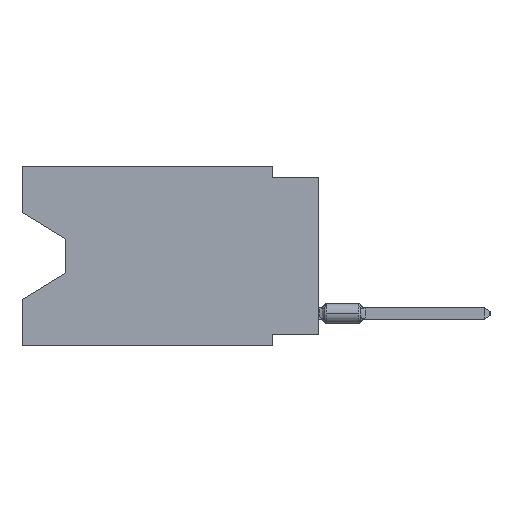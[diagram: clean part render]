
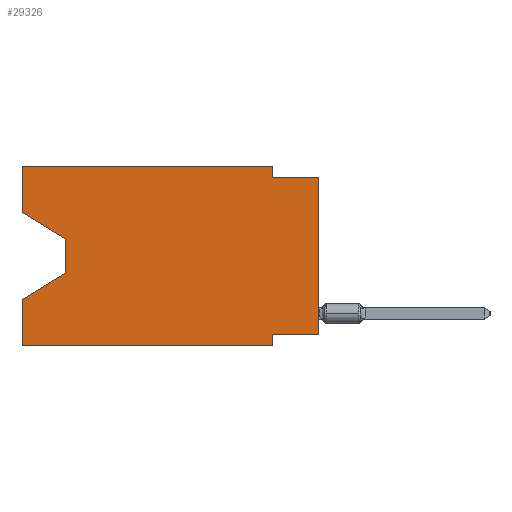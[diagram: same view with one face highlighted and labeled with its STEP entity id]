
A CAD part, left-side view. The second image highlights one B-rep face of the part: STEP entity #29326.
In plain terms, the highlighted planar face has unit normal (-1, 0, 0).
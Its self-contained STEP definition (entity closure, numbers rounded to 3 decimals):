
#378 = EDGE_CURVE ( 'NONE', #15556, #2593, #25521, .T. ) ;
#432 = CARTESIAN_POINT ( 'NONE',  ( 0., 2.54, 0. ) ) ;
#511 = ORIENTED_EDGE ( 'NONE', *, *, #27226, .F. ) ;
#1447 = DIRECTION ( 'NONE',  ( 0., 1., 0. ) ) ;
#1590 = DIRECTION ( 'NONE',  ( 0., 0., 1. ) ) ;
#1791 = DIRECTION ( 'NONE',  ( 0., -0.855, -0.519 ) ) ;
#1927 = CARTESIAN_POINT ( 'NONE',  ( 0., 2.54, -9.906 ) ) ;
#2593 = VERTEX_POINT ( 'NONE', #32092 ) ;
#2703 = VECTOR ( 'NONE', #1590, 1000. ) ;
#3058 = DIRECTION ( 'NONE',  ( 0., 0.855, -0.519 ) ) ;
#3186 = VERTEX_POINT ( 'NONE', #12722 ) ;
#3612 = EDGE_CURVE ( 'NONE', #22711, #16617, #22225, .T. ) ;
#4272 = DIRECTION ( 'NONE',  ( 1., 0., 0. ) ) ;
#4531 = CARTESIAN_POINT ( 'NONE',  ( 0., 0., 0. ) ) ;
#5199 = CARTESIAN_POINT ( 'NONE',  ( 0., 16.383, -7.36 ) ) ;
#5386 = DIRECTION ( 'NONE',  ( 0., 0., 1. ) ) ;
#5462 = DIRECTION ( 'NONE',  ( 0., -1., 0. ) ) ;
#5693 = DIRECTION ( 'NONE',  ( 0., -1., 0. ) ) ;
#6014 = LINE ( 'NONE', #6197, #28349 ) ;
#6197 = CARTESIAN_POINT ( 'NONE',  ( 0., 16.383, 0. ) ) ;
#6799 = EDGE_CURVE ( 'NONE', #3186, #20952, #14919, .T. ) ;
#7032 = FACE_OUTER_BOUND ( 'NONE', #18373, .T. ) ;
#7128 = ORIENTED_EDGE ( 'NONE', *, *, #35729, .T. ) ;
#7172 = ORIENTED_EDGE ( 'NONE', *, *, #3612, .T. ) ;
#7250 = CARTESIAN_POINT ( 'NONE',  ( 0., 2.54, 0. ) ) ;
#8237 = VERTEX_POINT ( 'NONE', #22842 ) ;
#8382 = LINE ( 'NONE', #17988, #21376 ) ;
#8900 = ORIENTED_EDGE ( 'NONE', *, *, #30977, .F. ) ;
#9232 = CARTESIAN_POINT ( 'NONE',  ( 0., 16.383, -9.906 ) ) ;
#9713 = ORIENTED_EDGE ( 'NONE', *, *, #31710, .F. ) ;
#11893 = VECTOR ( 'NONE', #5386, 1000. ) ;
#12301 = ORIENTED_EDGE ( 'NONE', *, *, #6799, .T. ) ;
#12355 = EDGE_CURVE ( 'NONE', #22711, #8237, #37967, .T. ) ;
#12722 = CARTESIAN_POINT ( 'NONE',  ( 0., 16.383, -9.906 ) ) ;
#13727 = CARTESIAN_POINT ( 'NONE',  ( 0., 16.383, -2.546 ) ) ;
#14317 = CARTESIAN_POINT ( 'NONE',  ( 0., 13.97, -4.013 ) ) ;
#14728 = CARTESIAN_POINT ( 'NONE',  ( 0., 13.97, -5.893 ) ) ;
#14842 = DIRECTION ( 'NONE',  ( 0., 0., 1. ) ) ;
#14919 = LINE ( 'NONE', #9232, #26796 ) ;
#15556 = VERTEX_POINT ( 'NONE', #432 ) ;
#15657 = VERTEX_POINT ( 'NONE', #13727 ) ;
#16235 = DIRECTION ( 'NONE',  ( 0., 0., -1. ) ) ;
#16363 = DIRECTION ( 'NONE',  ( 0., 0., -1. ) ) ;
#16617 = VERTEX_POINT ( 'NONE', #36670 ) ;
#16864 = EDGE_CURVE ( 'NONE', #15657, #26306, #34035, .T. ) ;
#17988 = CARTESIAN_POINT ( 'NONE',  ( 0., 13.97, -5.893 ) ) ;
#18373 = EDGE_LOOP ( 'NONE', ( #22738, #33115, #7128, #20148, #12301, #9713, #18782, #7172, #23808, #25670, #8900, #511 ) ) ;
#18782 = ORIENTED_EDGE ( 'NONE', *, *, #12355, .F. ) ;
#20148 = ORIENTED_EDGE ( 'NONE', *, *, #24530, .F. ) ;
#20176 = LINE ( 'NONE', #32192, #31609 ) ;
#20952 = VERTEX_POINT ( 'NONE', #1927 ) ;
#21231 = VECTOR ( 'NONE', #1791, 1000. ) ;
#21332 = VECTOR ( 'NONE', #16363, 1000. ) ;
#21376 = VECTOR ( 'NONE', #3058, 1000. ) ;
#21600 = LINE ( 'NONE', #34171, #30300 ) ;
#22225 = LINE ( 'NONE', #4531, #2703 ) ;
#22711 = VERTEX_POINT ( 'NONE', #27203 ) ;
#22738 = ORIENTED_EDGE ( 'NONE', *, *, #16864, .T. ) ;
#22842 = CARTESIAN_POINT ( 'NONE',  ( 0., 2.54, -9.271 ) ) ;
#23808 = ORIENTED_EDGE ( 'NONE', *, *, #28529, .F. ) ;
#24530 = EDGE_CURVE ( 'NONE', #3186, #37395, #31901, .T. ) ;
#24847 = DIRECTION ( 'NONE',  ( 0., 0., -1. ) ) ;
#24944 = DIRECTION ( 'NONE',  ( 0., -1., 0. ) ) ;
#25365 = EDGE_CURVE ( 'NONE', #26306, #30539, #25628, .T. ) ;
#25432 = LINE ( 'NONE', #37398, #36014 ) ;
#25521 = LINE ( 'NONE', #7250, #26675 ) ;
#25628 = LINE ( 'NONE', #28193, #21332 ) ;
#25670 = ORIENTED_EDGE ( 'NONE', *, *, #378, .F. ) ;
#25892 = PLANE ( 'NONE',  #31612 ) ;
#25920 = VECTOR ( 'NONE', #1447, 1000. ) ;
#26306 = VERTEX_POINT ( 'NONE', #14317 ) ;
#26675 = VECTOR ( 'NONE', #33767, 1000. ) ;
#26796 = VECTOR ( 'NONE', #5693, 1000. ) ;
#27203 = CARTESIAN_POINT ( 'NONE',  ( 0., 0., -9.271 ) ) ;
#27226 = EDGE_CURVE ( 'NONE', #15657, #35727, #6014, .T. ) ;
#28193 = CARTESIAN_POINT ( 'NONE',  ( 0., 13.97, -4.013 ) ) ;
#28349 = VECTOR ( 'NONE', #14842, 1000. ) ;
#28361 = CARTESIAN_POINT ( 'NONE',  ( 0., 0., -9.271 ) ) ;
#28529 = EDGE_CURVE ( 'NONE', #2593, #16617, #21600, .T. ) ;
#29326 = ADVANCED_FACE ( 'NONE', ( #7032 ), #25892, .F. ) ;
#30300 = VECTOR ( 'NONE', #24944, 1000. ) ;
#30539 = VERTEX_POINT ( 'NONE', #14728 ) ;
#30977 = EDGE_CURVE ( 'NONE', #35727, #15556, #20176, .T. ) ;
#31212 = CARTESIAN_POINT ( 'NONE',  ( 0., 16.383, 0. ) ) ;
#31471 = CARTESIAN_POINT ( 'NONE',  ( 0., 16.383, -2.546 ) ) ;
#31609 = VECTOR ( 'NONE', #5462, 1000. ) ;
#31612 = AXIS2_PLACEMENT_3D ( 'NONE', #31212, #4272, #16235 ) ;
#31710 = EDGE_CURVE ( 'NONE', #8237, #20952, #25432, .T. ) ;
#31901 = LINE ( 'NONE', #32316, #11893 ) ;
#32092 = CARTESIAN_POINT ( 'NONE',  ( 0., 2.54, -0.635 ) ) ;
#32192 = CARTESIAN_POINT ( 'NONE',  ( 0., 16.383, 0. ) ) ;
#32316 = CARTESIAN_POINT ( 'NONE',  ( 0., 16.383, 0. ) ) ;
#32541 = CARTESIAN_POINT ( 'NONE',  ( 0., 16.383, 0. ) ) ;
#33115 = ORIENTED_EDGE ( 'NONE', *, *, #25365, .T. ) ;
#33767 = DIRECTION ( 'NONE',  ( 0., 0., -1. ) ) ;
#34035 = LINE ( 'NONE', #31471, #21231 ) ;
#34171 = CARTESIAN_POINT ( 'NONE',  ( 0., 0., -0.635 ) ) ;
#35727 = VERTEX_POINT ( 'NONE', #32541 ) ;
#35729 = EDGE_CURVE ( 'NONE', #30539, #37395, #8382, .T. ) ;
#36014 = VECTOR ( 'NONE', #24847, 1000. ) ;
#36670 = CARTESIAN_POINT ( 'NONE',  ( 0., 0., -0.635 ) ) ;
#37395 = VERTEX_POINT ( 'NONE', #5199 ) ;
#37398 = CARTESIAN_POINT ( 'NONE',  ( 0., 2.54, -9.906 ) ) ;
#37967 = LINE ( 'NONE', #28361, #25920 ) ;
